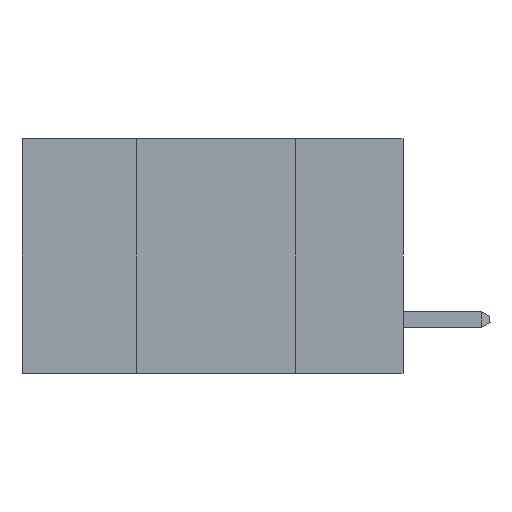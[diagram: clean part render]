
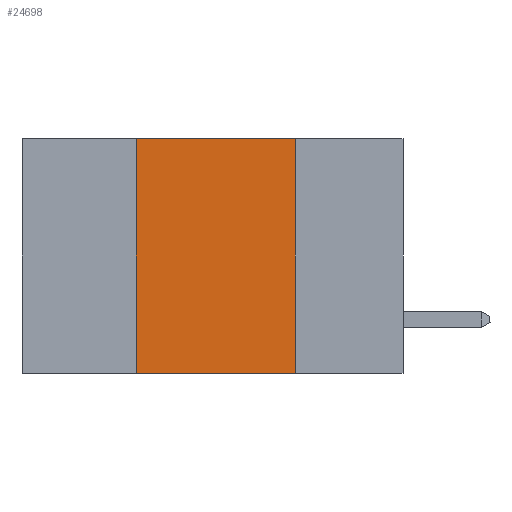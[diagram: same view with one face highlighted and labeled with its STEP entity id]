
A CAD part, left-side view. The second image highlights one B-rep face of the part: STEP entity #24698.
In plain terms, the highlighted planar face has unit normal (-1, 0, 0).
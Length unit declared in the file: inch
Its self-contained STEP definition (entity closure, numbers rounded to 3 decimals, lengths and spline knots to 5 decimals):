
#2829 = DIRECTION ( 'NONE',  ( 0., -1., 0. ) ) ;
#3858 = VERTEX_POINT ( 'NONE', #14895 ) ;
#4117 = DIRECTION ( 'NONE',  ( 0., -1., 0. ) ) ;
#5384 = FACE_OUTER_BOUND ( 'NONE', #14609, .T. ) ;
#6161 = ORIENTED_EDGE ( 'NONE', *, *, #43786, .F. ) ;
#6910 = DIRECTION ( 'NONE',  ( 0., 0., -1. ) ) ;
#10767 = EDGE_CURVE ( 'NONE', #29577, #3858, #39610, .T. ) ;
#12408 = CARTESIAN_POINT ( 'NONE',  ( 0., 0.17, 0. ) ) ;
#12861 = CARTESIAN_POINT ( 'NONE',  ( 0., 0.6, 0. ) ) ;
#14400 = EDGE_CURVE ( 'NONE', #35924, #46470, #46328, .T. ) ;
#14609 = EDGE_LOOP ( 'NONE', ( #29745, #6161, #27057, #26555 ) ) ;
#14895 = CARTESIAN_POINT ( 'NONE',  ( 0., 0.42, 0. ) ) ;
#17912 = CARTESIAN_POINT ( 'NONE',  ( 0., 0.6, -0.37 ) ) ;
#18389 = DIRECTION ( 'NONE',  ( 0., 0., 1. ) ) ;
#20838 = PLANE ( 'NONE',  #42720 ) ;
#24698 = ADVANCED_FACE ( 'NONE', ( #5384 ), #20838, .F. ) ;
#26555 = ORIENTED_EDGE ( 'NONE', *, *, #27481, .T. ) ;
#27006 = CARTESIAN_POINT ( 'NONE',  ( 0., 0.6, 0. ) ) ;
#27057 = ORIENTED_EDGE ( 'NONE', *, *, #10767, .F. ) ;
#27481 = EDGE_CURVE ( 'NONE', #29577, #46470, #45568, .T. ) ;
#27760 = CARTESIAN_POINT ( 'NONE',  ( 0., 0.42, -0.37 ) ) ;
#29577 = VERTEX_POINT ( 'NONE', #27760 ) ;
#29745 = ORIENTED_EDGE ( 'NONE', *, *, #14400, .F. ) ;
#33406 = CARTESIAN_POINT ( 'NONE',  ( 0., 0.17, 0. ) ) ;
#35807 = DIRECTION ( 'NONE',  ( 0., 0., -1. ) ) ;
#35924 = VERTEX_POINT ( 'NONE', #12408 ) ;
#39065 = VECTOR ( 'NONE', #6910, 39.37008 ) ;
#39610 = LINE ( 'NONE', #49779, #48694 ) ;
#40393 = VECTOR ( 'NONE', #4117, 39.37008 ) ;
#41072 = CARTESIAN_POINT ( 'NONE',  ( 0., 0.17, -0.37 ) ) ;
#41629 = LINE ( 'NONE', #27006, #40393 ) ;
#42720 = AXIS2_PLACEMENT_3D ( 'NONE', #12861, #47484, #35807 ) ;
#43786 = EDGE_CURVE ( 'NONE', #3858, #35924, #41629, .T. ) ;
#44370 = VECTOR ( 'NONE', #2829, 39.37008 ) ;
#45568 = LINE ( 'NONE', #17912, #44370 ) ;
#46328 = LINE ( 'NONE', #33406, #39065 ) ;
#46470 = VERTEX_POINT ( 'NONE', #41072 ) ;
#47484 = DIRECTION ( 'NONE',  ( 1., 0., 0. ) ) ;
#48694 = VECTOR ( 'NONE', #18389, 39.37008 ) ;
#49779 = CARTESIAN_POINT ( 'NONE',  ( 0., 0.42, 0. ) ) ;
